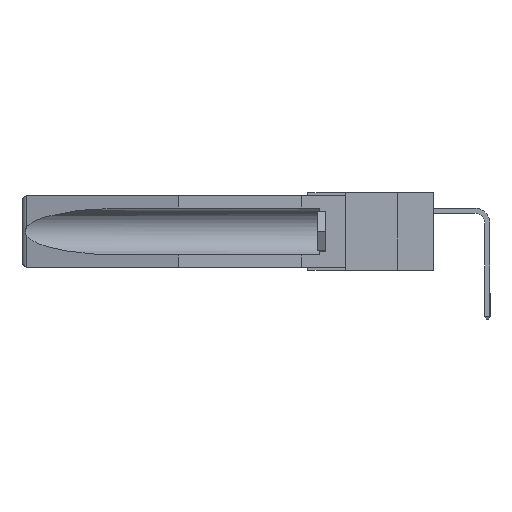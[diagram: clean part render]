
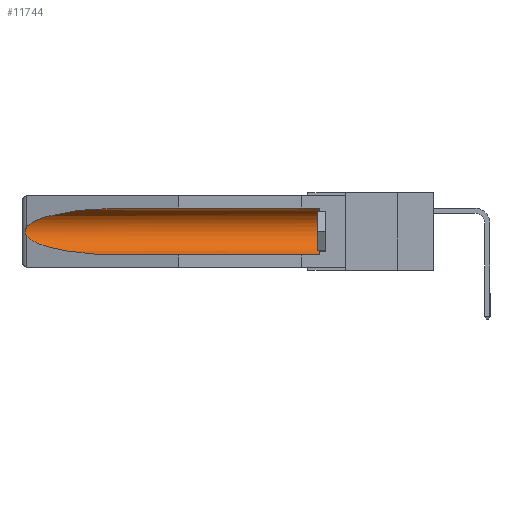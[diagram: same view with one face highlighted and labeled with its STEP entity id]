
A CAD part, left-side view. The second image highlights one B-rep face of the part: STEP entity #11744.
In plain terms, the highlighted cylindrical face has radius 2.857 mm (diameter 5.715 mm), a partial arc.
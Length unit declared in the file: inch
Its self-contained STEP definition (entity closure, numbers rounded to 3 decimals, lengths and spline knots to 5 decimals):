
#231 = VECTOR ( 'NONE', #7559, 39.37008 ) ;
#530 = CARTESIAN_POINT ( 'NONE',  ( 0.25451, 1.48313, -0.24835 ) ) ;
#543 = DIRECTION ( 'NONE',  ( 0., 0., 1. ) ) ;
#585 = CARTESIAN_POINT ( 'NONE',  ( 0.155, 0.126, -0.1715 ) ) ;
#894 = LINE ( 'NONE', #14503, #231 ) ;
#944 = CARTESIAN_POINT ( 'NONE',  ( 0.26597, 1.52961, -0.15275 ) ) ;
#1976 = DIRECTION ( 'NONE',  ( 0., 0., 1. ) ) ;
#2588 = ORIENTED_EDGE ( 'NONE', *, *, #12799, .T. ) ;
#2627 = CARTESIAN_POINT ( 'NONE',  ( 0.26597, 1.5296, -0.19026 ) ) ;
#2683 = CARTESIAN_POINT ( 'NONE',  ( 0.26655, 1.53094, -0.18657 ) ) ;
#2815 = EDGE_CURVE ( 'NONE', #8053, #9114, #17634, .T. ) ;
#3913 = CARTESIAN_POINT ( 'NONE',  ( 0.2675, 1.53308, -0.16763 ) ) ;
#4703 = CARTESIAN_POINT ( 'NONE',  ( 0.26537, 1.52718, -0.19328 ) ) ;
#4783 = VECTOR ( 'NONE', #8399, 39.37008 ) ;
#4813 = CARTESIAN_POINT ( 'NONE',  ( 0.21114, 1.30732, -0.284 ) ) ;
#4887 = CARTESIAN_POINT ( 'NONE',  ( 0.155, -0.30754, -0.1715 ) ) ;
#5037 = CARTESIAN_POINT ( 'NONE',  ( 0.155, 1.07973, -0.059 ) ) ;
#5044 = CARTESIAN_POINT ( 'NONE',  ( 0.26537, 1.52718, -0.14972 ) ) ;
#5311 =( BOUNDED_CURVE ( )  B_SPLINE_CURVE ( 3, ( #6043, #14373, #7347, #11475 ),
 .UNSPECIFIED., .F., .F. ) 
 B_SPLINE_CURVE_WITH_KNOTS ( ( 4, 4 ),
 ( 4.71239, 6.08839 ),
 .UNSPECIFIED. ) 
 CURVE ( )  GEOMETRIC_REPRESENTATION_ITEM ( )  RATIONAL_B_SPLINE_CURVE ( ( 1., 0.848, 0.848, 1. ) ) 
 REPRESENTATION_ITEM ( '' )  );
#6043 = CARTESIAN_POINT ( 'NONE',  ( 0.155, 1.07973, -0.059 ) ) ;
#6669 = EDGE_LOOP ( 'NONE', ( #16991, #17443, #6695, #14235, #14341, #2588 ) ) ;
#6695 = ORIENTED_EDGE ( 'NONE', *, *, #2815, .T. ) ;
#7347 = CARTESIAN_POINT ( 'NONE',  ( 0.25451, 1.48313, -0.09465 ) ) ;
#7559 = DIRECTION ( 'NONE',  ( 0., 1., 0. ) ) ;
#8053 = VERTEX_POINT ( 'NONE', #14754 ) ;
#8070 = CARTESIAN_POINT ( 'NONE',  ( 0.26537, 1.52718, -0.19328 ) ) ;
#8243 = CARTESIAN_POINT ( 'NONE',  ( 0.26654, 1.53092, -0.15636 ) ) ;
#8399 = DIRECTION ( 'NONE',  ( 0., 1., 0. ) ) ;
#8473 = LINE ( 'NONE', #14004, #4783 ) ;
#8834 = DIRECTION ( 'NONE',  ( 0., 1., 0. ) ) ;
#9114 = VERTEX_POINT ( 'NONE', #9495 ) ;
#9333 = CARTESIAN_POINT ( 'NONE',  ( 0.155, 0.126, -0.284 ) ) ;
#9495 = CARTESIAN_POINT ( 'NONE',  ( 0.155, 1.07973, -0.284 ) ) ;
#10654 = CARTESIAN_POINT ( 'NONE',  ( 0.155, 1.07973, -0.284 ) ) ;
#10826 = CARTESIAN_POINT ( 'NONE',  ( 0.2675, 1.53308, -0.17534 ) ) ;
#11027 = CARTESIAN_POINT ( 'NONE',  ( 0.155, 0.126, -0.059 ) ) ;
#11261 = VERTEX_POINT ( 'NONE', #13196 ) ;
#11475 = CARTESIAN_POINT ( 'NONE',  ( 0.26537, 1.52718, -0.14972 ) ) ;
#11731 = AXIS2_PLACEMENT_3D ( 'NONE', #585, #11804, #1976 ) ;
#11744 = ADVANCED_FACE ( 'NONE', ( #12392 ), #15398, .F. ) ;
#11804 = DIRECTION ( 'NONE',  ( 0., -1., 0. ) ) ;
#12132 = VERTEX_POINT ( 'NONE', #11027 ) ;
#12392 = FACE_OUTER_BOUND ( 'NONE', #6669, .T. ) ;
#12799 = EDGE_CURVE ( 'NONE', #12132, #13128, #894, .T. ) ;
#13128 = VERTEX_POINT ( 'NONE', #5037 ) ;
#13196 = CARTESIAN_POINT ( 'NONE',  ( 0.26537, 1.52718, -0.14972 ) ) ;
#13308 = VERTEX_POINT ( 'NONE', #9333 ) ;
#14004 = CARTESIAN_POINT ( 'NONE',  ( 0.155, -0.30754, -0.284 ) ) ;
#14055 = CIRCLE ( 'NONE', #11731, 0.1125 ) ;
#14235 = ORIENTED_EDGE ( 'NONE', *, *, #14419, .F. ) ;
#14341 = ORIENTED_EDGE ( 'NONE', *, *, #17057, .T. ) ;
#14373 = CARTESIAN_POINT ( 'NONE',  ( 0.21114, 1.30732, -0.059 ) ) ;
#14419 = EDGE_CURVE ( 'NONE', #13308, #9114, #8473, .T. ) ;
#14503 = CARTESIAN_POINT ( 'NONE',  ( 0.155, -0.30754, -0.059 ) ) ;
#14754 = CARTESIAN_POINT ( 'NONE',  ( 0.26537, 1.52718, -0.19328 ) ) ;
#15398 = CYLINDRICAL_SURFACE ( 'NONE', #15691, 0.1125 ) ;
#15532 = B_SPLINE_CURVE_WITH_KNOTS ( 'NONE', 3,
 ( #5044, #944, #8243, #17812, #3913, #10826, #16363, #2683, #2627, #8070 ),
 .UNSPECIFIED., .F., .F.,
 ( 4, 2, 2, 2, 4 ),
 ( 0., 0.00029, 0.00058, 0.00087, 0.00117 ),
 .UNSPECIFIED. ) ;
#15691 = AXIS2_PLACEMENT_3D ( 'NONE', #4887, #8834, #543 ) ;
#15803 = EDGE_CURVE ( 'NONE', #13128, #11261, #5311, .T. ) ;
#16363 = CARTESIAN_POINT ( 'NONE',  ( 0.2673, 1.53269, -0.17917 ) ) ;
#16991 = ORIENTED_EDGE ( 'NONE', *, *, #15803, .T. ) ;
#17057 = EDGE_CURVE ( 'NONE', #13308, #12132, #14055, .T. ) ;
#17443 = ORIENTED_EDGE ( 'NONE', *, *, #17570, .T. ) ;
#17570 = EDGE_CURVE ( 'NONE', #11261, #8053, #15532, .T. ) ;
#17634 =( BOUNDED_CURVE ( )  B_SPLINE_CURVE ( 3, ( #4703, #530, #4813, #10654 ),
 .UNSPECIFIED., .F., .F. ) 
 B_SPLINE_CURVE_WITH_KNOTS ( ( 4, 4 ),
 ( 0.1948, 1.5708 ),
 .UNSPECIFIED. ) 
 CURVE ( )  GEOMETRIC_REPRESENTATION_ITEM ( )  RATIONAL_B_SPLINE_CURVE ( ( 1., 0.848, 0.848, 1. ) ) 
 REPRESENTATION_ITEM ( '' )  );
#17812 = CARTESIAN_POINT ( 'NONE',  ( 0.2673, 1.5327, -0.16383 ) ) ;
